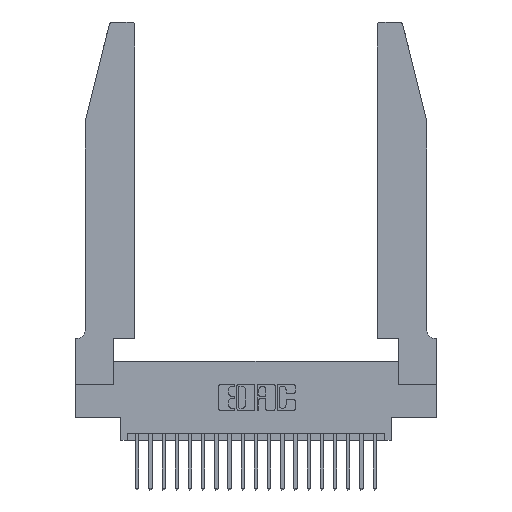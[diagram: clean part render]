
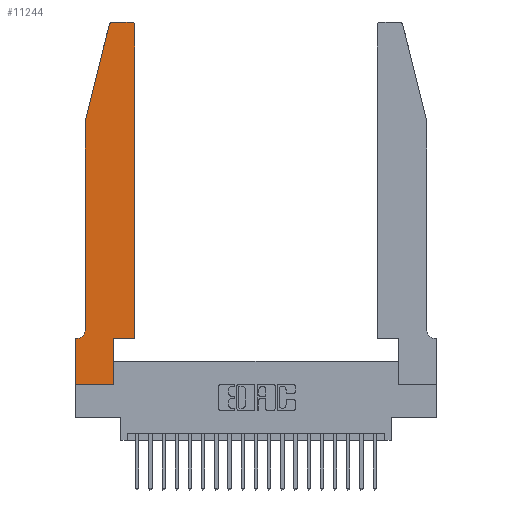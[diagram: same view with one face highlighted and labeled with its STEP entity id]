
A CAD part, top view. The second image highlights one B-rep face of the part: STEP entity #11244.
In plain terms, the highlighted planar face has unit normal (0, 0, 1).
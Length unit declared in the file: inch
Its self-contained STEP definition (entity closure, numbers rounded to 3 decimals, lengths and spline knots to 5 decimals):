
#66 = CARTESIAN_POINT ( 'NONE',  ( 0.4505, 2.72, 0.37 ) ) ;
#385 = ORIENTED_EDGE ( 'NONE', *, *, #18883, .T. ) ;
#620 = DIRECTION ( 'NONE',  ( -0.239, -0.971, 0. ) ) ;
#657 = VERTEX_POINT ( 'NONE', #17001 ) ;
#1085 = EDGE_LOOP ( 'NONE', ( #4098, #15054, #12379, #385, #8786, #6039, #13879, #4593, #7192, #4452, #19421, #10715 ) ) ;
#1189 = LINE ( 'NONE', #22263, #10075 ) ;
#1490 = EDGE_CURVE ( 'NONE', #4464, #8327, #12868, .T. ) ;
#1856 = EDGE_CURVE ( 'NONE', #13407, #20934, #5081, .T. ) ;
#2072 = AXIS2_PLACEMENT_3D ( 'NONE', #15275, #20462, #8055 ) ;
#2113 = VERTEX_POINT ( 'NONE', #66 ) ;
#3503 = CARTESIAN_POINT ( 'NONE',  ( 0.0755, 2., 0.37 ) ) ;
#3828 = VECTOR ( 'NONE', #9556, 39.37008 ) ;
#4098 = ORIENTED_EDGE ( 'NONE', *, *, #9024, .T. ) ;
#4104 = DIRECTION ( 'NONE',  ( 0., 1., 0. ) ) ;
#4358 = CARTESIAN_POINT ( 'NONE',  ( 0.0055, 0.35, 0.37 ) ) ;
#4452 = ORIENTED_EDGE ( 'NONE', *, *, #4516, .T. ) ;
#4464 = VERTEX_POINT ( 'NONE', #4358 ) ;
#4516 = EDGE_CURVE ( 'NONE', #11143, #657, #4655, .T. ) ;
#4593 = ORIENTED_EDGE ( 'NONE', *, *, #1856, .T. ) ;
#4655 = LINE ( 'NONE', #22027, #3828 ) ;
#4886 = LINE ( 'NONE', #21856, #12354 ) ;
#5081 = LINE ( 'NONE', #5991, #6755 ) ;
#5501 = VERTEX_POINT ( 'NONE', #10874 ) ;
#5936 = CARTESIAN_POINT ( 'NONE',  ( 0.4205, 2.75, 0.37 ) ) ;
#5979 = VERTEX_POINT ( 'NONE', #5936 ) ;
#5991 = CARTESIAN_POINT ( 'NONE',  ( 0., 0., 0.37 ) ) ;
#6039 = ORIENTED_EDGE ( 'NONE', *, *, #1490, .T. ) ;
#6619 = FACE_OUTER_BOUND ( 'NONE', #1085, .T. ) ;
#6666 = EDGE_CURVE ( 'NONE', #11364, #19990, #4886, .T. ) ;
#6755 = VECTOR ( 'NONE', #13424, 39.37008 ) ;
#7192 = ORIENTED_EDGE ( 'NONE', *, *, #15042, .T. ) ;
#7514 = CARTESIAN_POINT ( 'NONE',  ( 0.0055, 0.42, 0.37 ) ) ;
#7727 = AXIS2_PLACEMENT_3D ( 'NONE', #20053, #11128, #21906 ) ;
#7750 = CARTESIAN_POINT ( 'NONE',  ( 0.4505, 0.35, 0.37 ) ) ;
#8055 = DIRECTION ( 'NONE',  ( 1., 0., 0. ) ) ;
#8061 = VECTOR ( 'NONE', #10218, 39.37008 ) ;
#8327 = VERTEX_POINT ( 'NONE', #14738 ) ;
#8786 = ORIENTED_EDGE ( 'NONE', *, *, #12222, .T. ) ;
#9024 = EDGE_CURVE ( 'NONE', #5979, #5501, #15854, .T. ) ;
#9059 = CARTESIAN_POINT ( 'NONE',  ( 0.0755, 2., 0.37 ) ) ;
#9556 = DIRECTION ( 'NONE',  ( 1., 0., 0. ) ) ;
#9583 = CARTESIAN_POINT ( 'NONE',  ( 0.25487, 2.72718, 0.37 ) ) ;
#10075 = VECTOR ( 'NONE', #17110, 39.37008 ) ;
#10218 = DIRECTION ( 'NONE',  ( -1., 0., 0. ) ) ;
#10715 = ORIENTED_EDGE ( 'NONE', *, *, #20746, .T. ) ;
#10768 = DIRECTION ( 'NONE',  ( 0., 0., -1. ) ) ;
#10874 = CARTESIAN_POINT ( 'NONE',  ( 0.284, 2.75, 0.37 ) ) ;
#11128 = DIRECTION ( 'NONE',  ( 0., 0., 1. ) ) ;
#11143 = VERTEX_POINT ( 'NONE', #21375 ) ;
#11244 = ADVANCED_FACE ( 'NONE', ( #6619 ), #12773, .T. ) ;
#11276 = CIRCLE ( 'NONE', #2072, 0.03 ) ;
#11364 = VERTEX_POINT ( 'NONE', #9583 ) ;
#11753 = CIRCLE ( 'NONE', #16030, 0.03 ) ;
#11802 = CARTESIAN_POINT ( 'NONE',  ( 0., 0., 0.37 ) ) ;
#12222 = EDGE_CURVE ( 'NONE', #20672, #4464, #22078, .T. ) ;
#12354 = VECTOR ( 'NONE', #620, 39.37008 ) ;
#12379 = ORIENTED_EDGE ( 'NONE', *, *, #6666, .T. ) ;
#12489 = EDGE_CURVE ( 'NONE', #5501, #11364, #11276, .T. ) ;
#12603 = CARTESIAN_POINT ( 'NONE',  ( 0.4205, 2.72, 0.37 ) ) ;
#12773 = PLANE ( 'NONE',  #7727 ) ;
#12868 = LINE ( 'NONE', #16449, #17030 ) ;
#13407 = VERTEX_POINT ( 'NONE', #16024 ) ;
#13424 = DIRECTION ( 'NONE',  ( 1., 0., 0. ) ) ;
#13871 = CARTESIAN_POINT ( 'NONE',  ( 0.0755, 0.42, 0.37 ) ) ;
#13879 = ORIENTED_EDGE ( 'NONE', *, *, #21090, .T. ) ;
#13882 = CARTESIAN_POINT ( 'NONE',  ( 0.2605, 2.75, 0.37 ) ) ;
#14230 = EDGE_CURVE ( 'NONE', #657, #2113, #22266, .T. ) ;
#14738 = CARTESIAN_POINT ( 'NONE',  ( 0., 0.35, 0.37 ) ) ;
#15041 = DIRECTION ( 'NONE',  ( -1., 0., 0. ) ) ;
#15042 = EDGE_CURVE ( 'NONE', #20934, #11143, #1189, .T. ) ;
#15054 = ORIENTED_EDGE ( 'NONE', *, *, #12489, .T. ) ;
#15275 = CARTESIAN_POINT ( 'NONE',  ( 0.284, 2.72, 0.37 ) ) ;
#15854 = LINE ( 'NONE', #13882, #8061 ) ;
#16004 = LINE ( 'NONE', #9059, #19583 ) ;
#16024 = CARTESIAN_POINT ( 'NONE',  ( 0., 0., 0.37 ) ) ;
#16030 = AXIS2_PLACEMENT_3D ( 'NONE', #12603, #21288, #21208 ) ;
#16449 = CARTESIAN_POINT ( 'NONE',  ( 0.0755, 0.35, 0.37 ) ) ;
#17001 = CARTESIAN_POINT ( 'NONE',  ( 0.4505, 0.35, 0.37 ) ) ;
#17030 = VECTOR ( 'NONE', #15041, 39.37008 ) ;
#17110 = DIRECTION ( 'NONE',  ( 0., 1., 0. ) ) ;
#17178 = DIRECTION ( 'NONE',  ( 0., -1., 0. ) ) ;
#18883 = EDGE_CURVE ( 'NONE', #19990, #20672, #16004, .T. ) ;
#19246 = VECTOR ( 'NONE', #4104, 39.37008 ) ;
#19421 = ORIENTED_EDGE ( 'NONE', *, *, #14230, .T. ) ;
#19583 = VECTOR ( 'NONE', #21460, 39.37008 ) ;
#19614 = DIRECTION ( 'NONE',  ( -1., 0., 0. ) ) ;
#19728 = CARTESIAN_POINT ( 'NONE',  ( 0.2865, 0., 0.37 ) ) ;
#19990 = VERTEX_POINT ( 'NONE', #3503 ) ;
#20053 = CARTESIAN_POINT ( 'NONE',  ( 0., 0.35, 0.37 ) ) ;
#20351 = LINE ( 'NONE', #11802, #22008 ) ;
#20462 = DIRECTION ( 'NONE',  ( 0., 0., 1. ) ) ;
#20661 = AXIS2_PLACEMENT_3D ( 'NONE', #7514, #10768, #19614 ) ;
#20672 = VERTEX_POINT ( 'NONE', #13871 ) ;
#20746 = EDGE_CURVE ( 'NONE', #2113, #5979, #11753, .T. ) ;
#20934 = VERTEX_POINT ( 'NONE', #19728 ) ;
#21090 = EDGE_CURVE ( 'NONE', #8327, #13407, #20351, .T. ) ;
#21208 = DIRECTION ( 'NONE',  ( 1., 0., 0. ) ) ;
#21288 = DIRECTION ( 'NONE',  ( 0., 0., 1. ) ) ;
#21375 = CARTESIAN_POINT ( 'NONE',  ( 0.2865, 0.35, 0.37 ) ) ;
#21460 = DIRECTION ( 'NONE',  ( 0., -1., 0. ) ) ;
#21856 = CARTESIAN_POINT ( 'NONE',  ( 0.0755, 2., 0.37 ) ) ;
#21906 = DIRECTION ( 'NONE',  ( 1., 0., 0. ) ) ;
#22008 = VECTOR ( 'NONE', #17178, 39.37008 ) ;
#22027 = CARTESIAN_POINT ( 'NONE',  ( 0.4505, 0.35, 0.37 ) ) ;
#22078 = CIRCLE ( 'NONE', #20661, 0.07 ) ;
#22263 = CARTESIAN_POINT ( 'NONE',  ( 0.2865, 0.35, 0.37 ) ) ;
#22266 = LINE ( 'NONE', #7750, #19246 ) ;
